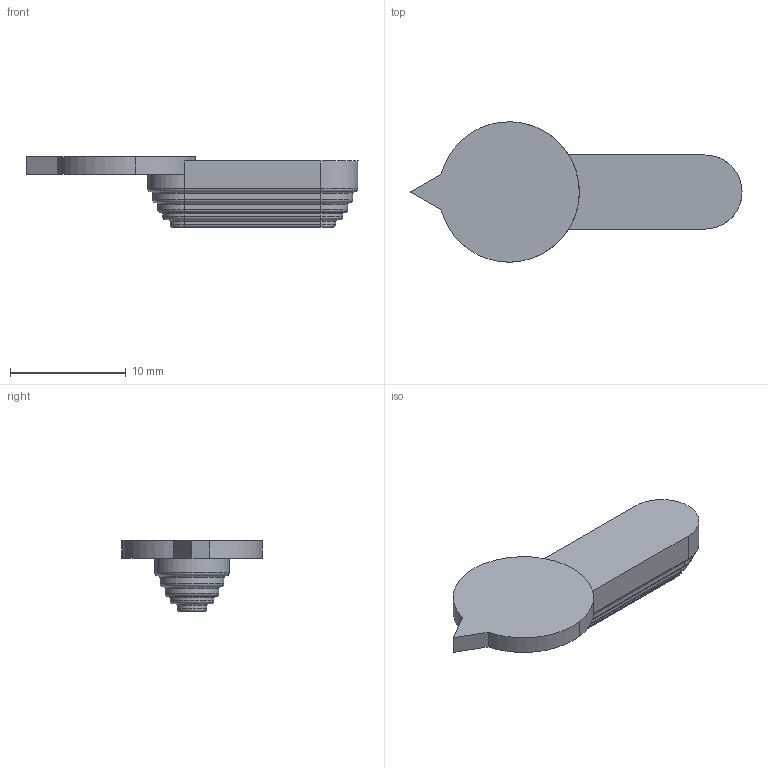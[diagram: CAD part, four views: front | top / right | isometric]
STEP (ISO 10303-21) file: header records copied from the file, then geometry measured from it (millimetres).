
FILE_DESCRIPTION((''),'2;1');
FILE_NAME('SOLID4','2019-01-20T17:52:54',('Cust'),(''),'CREO PARAMETRIC BY PTC INC, 2018300','CREO PARAMETRIC BY PTC INC, 2018300','');
FILE_SCHEMA(('AUTOMOTIVE_DESIGN { 1 0 10303 214 1 1 1 1 }'));
Length unit declared in the file: inch
Products named in the file (1): SOLID4
Bounding box: 28.66 x 12.13 x 6.12 mm (x, y, z)
Volume: 648 mm3; surface area: 658.8 mm2
Topology: 1 solids, 1 shells, 69 faces, 157 edges, 94 vertices
Faces by surface type: cylinder 27, plane 20, torus 13, bspline 5, extrusion 4
Entity records: 4079 total; most frequent: CARTESIAN_POINT 1966, DIRECTION 343, ORIENTED_EDGE 314, PRESENTATION_STYLE_ASSIGNMENT 158, STYLED_ITEM 158, CURVE_STYLE 157, EDGE_CURVE 157, AXIS2_PLACEMENT_3D 135
